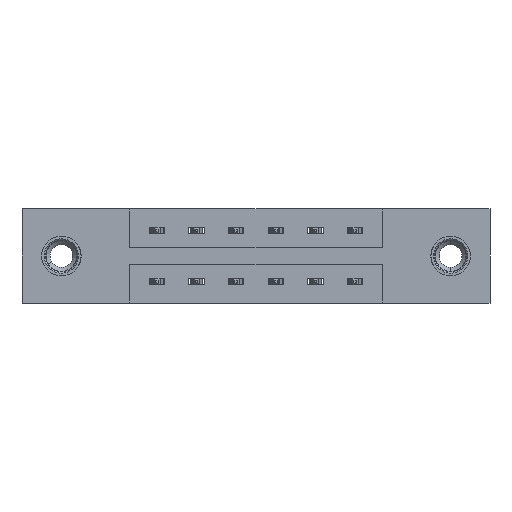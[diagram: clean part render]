
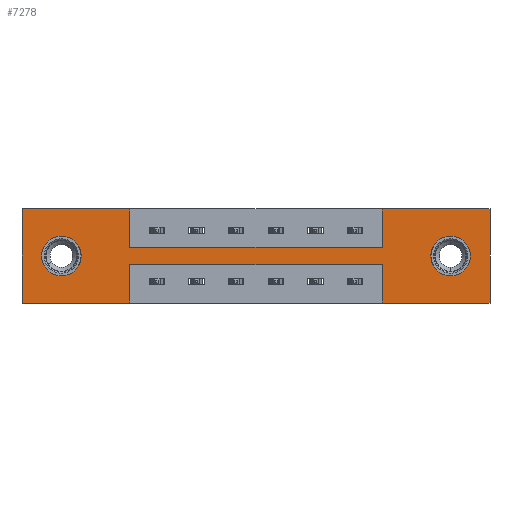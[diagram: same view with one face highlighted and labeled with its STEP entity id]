
A CAD part, front view. The second image highlights one B-rep face of the part: STEP entity #7278.
In plain terms, the highlighted planar face has unit normal (0, -1, 0).
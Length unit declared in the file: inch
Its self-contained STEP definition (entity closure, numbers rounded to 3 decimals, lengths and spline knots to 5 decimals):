
#63 = FACE_BOUND ( 'NONE', #5613, .T. ) ;
#370 = DIRECTION ( 'NONE',  ( 0., 0., 1. ) ) ;
#377 = DIRECTION ( 'NONE',  ( 0., 0., 1. ) ) ;
#444 = DIRECTION ( 'NONE',  ( 0., 0., 1. ) ) ;
#458 = CARTESIAN_POINT ( 'NONE',  ( 0., 0., 0. ) ) ;
#507 = DIRECTION ( 'NONE',  ( 0., 0., 1. ) ) ;
#726 = LINE ( 'NONE', #10218, #7876 ) ;
#745 = CARTESIAN_POINT ( 'NONE',  ( 0., 0., 0. ) ) ;
#850 = EDGE_CURVE ( 'NONE', #5885, #9751, #726, .T. ) ;
#932 = LINE ( 'NONE', #745, #8603 ) ;
#1276 = LINE ( 'NONE', #458, #6536 ) ;
#1487 = EDGE_LOOP ( 'NONE', ( #7969, #8581, #2194, #3082, #7238, #6173, #7760, #5779, #2649, #6108, #7598, #5105 ) ) ;
#1727 = DIRECTION ( 'NONE',  ( 0., 1., 0. ) ) ;
#1760 = DIRECTION ( 'NONE',  ( -1., 0., 0. ) ) ;
#1803 = CARTESIAN_POINT ( 'NONE',  ( 1.842, 0., -0.37 ) ) ;
#1879 = EDGE_CURVE ( 'NONE', #3260, #9909, #4144, .T. ) ;
#1984 = DIRECTION ( 'NONE',  ( 0., 0., -1. ) ) ;
#1999 = ORIENTED_EDGE ( 'NONE', *, *, #6703, .T. ) ;
#2004 = AXIS2_PLACEMENT_3D ( 'NONE', #3035, #6386, #4793 ) ;
#2066 = EDGE_CURVE ( 'NONE', #6498, #4784, #5661, .T. ) ;
#2078 = FACE_BOUND ( 'NONE', #5520, .T. ) ;
#2093 = DIRECTION ( 'NONE',  ( 0., 0., -1. ) ) ;
#2112 = VERTEX_POINT ( 'NONE', #7052 ) ;
#2194 = ORIENTED_EDGE ( 'NONE', *, *, #6583, .F. ) ;
#2346 = EDGE_CURVE ( 'NONE', #5500, #9208, #4010, .T. ) ;
#2453 = EDGE_CURVE ( 'NONE', #5859, #4353, #932, .T. ) ;
#2478 = LINE ( 'NONE', #4510, #4418 ) ;
#2520 = CARTESIAN_POINT ( 'NONE',  ( 1.417, 0., -0.22 ) ) ;
#2649 = ORIENTED_EDGE ( 'NONE', *, *, #8622, .F. ) ;
#2692 = DIRECTION ( 'NONE',  ( 0., 0., -1. ) ) ;
#2848 = DIRECTION ( 'NONE',  ( 0., 1., 0. ) ) ;
#3035 = CARTESIAN_POINT ( 'NONE',  ( 0.155, 0., -0.185 ) ) ;
#3072 = DIRECTION ( 'NONE',  ( 0., 1., 0. ) ) ;
#3082 = ORIENTED_EDGE ( 'NONE', *, *, #1879, .F. ) ;
#3260 = VERTEX_POINT ( 'NONE', #1803 ) ;
#3330 = CARTESIAN_POINT ( 'NONE',  ( 1.687, 0., -0.185 ) ) ;
#3487 = LINE ( 'NONE', #3675, #8743 ) ;
#3525 = CARTESIAN_POINT ( 'NONE',  ( 0.155, 0., -0.185 ) ) ;
#3571 = CARTESIAN_POINT ( 'NONE',  ( 0., 0., 0. ) ) ;
#3597 = CARTESIAN_POINT ( 'NONE',  ( 1.417, 0., -0.37 ) ) ;
#3664 = DIRECTION ( 'NONE',  ( 1., 0., 0. ) ) ;
#3675 = CARTESIAN_POINT ( 'NONE',  ( 1.417, 0., 0. ) ) ;
#3828 = DIRECTION ( 'NONE',  ( 0., 0., -1. ) ) ;
#3837 = CARTESIAN_POINT ( 'NONE',  ( 0.155, 0., -0.263 ) ) ;
#3886 = FACE_OUTER_BOUND ( 'NONE', #1487, .T. ) ;
#3925 = VERTEX_POINT ( 'NONE', #8525 ) ;
#3940 = EDGE_CURVE ( 'NONE', #8031, #3925, #1276, .T. ) ;
#4006 = VECTOR ( 'NONE', #6531, 39.37008 ) ;
#4010 = CIRCLE ( 'NONE', #5925, 0.078 ) ;
#4053 = CARTESIAN_POINT ( 'NONE',  ( 0.425, 0., -0.37 ) ) ;
#4144 = LINE ( 'NONE', #6759, #10363 ) ;
#4169 = CARTESIAN_POINT ( 'NONE',  ( 1.687, 0., -0.263 ) ) ;
#4216 = VECTOR ( 'NONE', #377, 39.37008 ) ;
#4353 = VERTEX_POINT ( 'NONE', #5082 ) ;
#4418 = VECTOR ( 'NONE', #2093, 39.37008 ) ;
#4470 = EDGE_CURVE ( 'NONE', #9751, #5859, #6525, .T. ) ;
#4497 = CARTESIAN_POINT ( 'NONE',  ( 0.425, 0., -0.22 ) ) ;
#4510 = CARTESIAN_POINT ( 'NONE',  ( 0.425, 0., -0.37 ) ) ;
#4784 = VERTEX_POINT ( 'NONE', #6751 ) ;
#4793 = DIRECTION ( 'NONE',  ( 0., 0., 1. ) ) ;
#5082 = CARTESIAN_POINT ( 'NONE',  ( 0.425, 0., 0. ) ) ;
#5105 = ORIENTED_EDGE ( 'NONE', *, *, #850, .F. ) ;
#5111 = DIRECTION ( 'NONE',  ( 1., 0., 0. ) ) ;
#5251 = CARTESIAN_POINT ( 'NONE',  ( 1.687, 0., -0.107 ) ) ;
#5297 = DIRECTION ( 'NONE',  ( -1., 0., 0. ) ) ;
#5389 = CARTESIAN_POINT ( 'NONE',  ( 0.425, 0., -0.15 ) ) ;
#5396 = DIRECTION ( 'NONE',  ( -1., 0., 0. ) ) ;
#5412 = LINE ( 'NONE', #7024, #7847 ) ;
#5500 = VERTEX_POINT ( 'NONE', #5251 ) ;
#5520 = EDGE_LOOP ( 'NONE', ( #7944, #1999 ) ) ;
#5613 = EDGE_LOOP ( 'NONE', ( #9435, #9003 ) ) ;
#5646 = CARTESIAN_POINT ( 'NONE',  ( 0., 0., 0. ) ) ;
#5661 = LINE ( 'NONE', #4497, #9735 ) ;
#5779 = ORIENTED_EDGE ( 'NONE', *, *, #6575, .F. ) ;
#5794 = VERTEX_POINT ( 'NONE', #3837 ) ;
#5810 = CARTESIAN_POINT ( 'NONE',  ( 0., 0., -0.37 ) ) ;
#5859 = VERTEX_POINT ( 'NONE', #5646 ) ;
#5885 = VERTEX_POINT ( 'NONE', #4053 ) ;
#5925 = AXIS2_PLACEMENT_3D ( 'NONE', #3330, #1727, #2692 ) ;
#6108 = ORIENTED_EDGE ( 'NONE', *, *, #2453, .F. ) ;
#6166 = AXIS2_PLACEMENT_3D ( 'NONE', #7216, #3072, #8852 ) ;
#6173 = ORIENTED_EDGE ( 'NONE', *, *, #3940, .F. ) ;
#6213 = LINE ( 'NONE', #9437, #9136 ) ;
#6254 = EDGE_CURVE ( 'NONE', #4784, #5885, #2478, .T. ) ;
#6333 = LINE ( 'NONE', #5389, #8882 ) ;
#6386 = DIRECTION ( 'NONE',  ( 0., 1., 0. ) ) ;
#6498 = VERTEX_POINT ( 'NONE', #2520 ) ;
#6525 = LINE ( 'NONE', #3571, #4216 ) ;
#6531 = DIRECTION ( 'NONE',  ( 0., 0., -1. ) ) ;
#6536 = VECTOR ( 'NONE', #10277, 39.37008 ) ;
#6575 = EDGE_CURVE ( 'NONE', #2112, #8388, #6333, .T. ) ;
#6583 = EDGE_CURVE ( 'NONE', #9909, #6498, #6213, .T. ) ;
#6703 = EDGE_CURVE ( 'NONE', #5794, #8820, #6734, .T. ) ;
#6734 = CIRCLE ( 'NONE', #2004, 0.078 ) ;
#6751 = CARTESIAN_POINT ( 'NONE',  ( 0.425, 0., -0.22 ) ) ;
#6759 = CARTESIAN_POINT ( 'NONE',  ( 0., 0., -0.37 ) ) ;
#7024 = CARTESIAN_POINT ( 'NONE',  ( 0.425, 0., 0. ) ) ;
#7052 = CARTESIAN_POINT ( 'NONE',  ( 0.425, 0., -0.15 ) ) ;
#7216 = CARTESIAN_POINT ( 'NONE',  ( 1.687, 0., -0.185 ) ) ;
#7238 = ORIENTED_EDGE ( 'NONE', *, *, #7986, .F. ) ;
#7278 = ADVANCED_FACE ( 'NONE', ( #63, #2078, #3886 ), #9481, .T. ) ;
#7297 = CIRCLE ( 'NONE', #6166, 0.078 ) ;
#7305 = LINE ( 'NONE', #9634, #4006 ) ;
#7502 = CARTESIAN_POINT ( 'NONE',  ( 0.155, 0., -0.107 ) ) ;
#7564 = EDGE_CURVE ( 'NONE', #8388, #8031, #3487, .T. ) ;
#7598 = ORIENTED_EDGE ( 'NONE', *, *, #4470, .F. ) ;
#7760 = ORIENTED_EDGE ( 'NONE', *, *, #7564, .F. ) ;
#7800 = AXIS2_PLACEMENT_3D ( 'NONE', #9427, #7917, #3828 ) ;
#7847 = VECTOR ( 'NONE', #1984, 39.37008 ) ;
#7872 = CARTESIAN_POINT ( 'NONE',  ( 1.417, 0., -0.15 ) ) ;
#7876 = VECTOR ( 'NONE', #5297, 39.37008 ) ;
#7917 = DIRECTION ( 'NONE',  ( 0., -1., 0. ) ) ;
#7944 = ORIENTED_EDGE ( 'NONE', *, *, #9924, .T. ) ;
#7969 = ORIENTED_EDGE ( 'NONE', *, *, #6254, .F. ) ;
#7986 = EDGE_CURVE ( 'NONE', #3925, #3260, #7305, .T. ) ;
#8031 = VERTEX_POINT ( 'NONE', #10506 ) ;
#8355 = AXIS2_PLACEMENT_3D ( 'NONE', #3525, #2848, #370 ) ;
#8388 = VERTEX_POINT ( 'NONE', #7872 ) ;
#8412 = CIRCLE ( 'NONE', #8355, 0.078 ) ;
#8525 = CARTESIAN_POINT ( 'NONE',  ( 1.842, 0., 0. ) ) ;
#8581 = ORIENTED_EDGE ( 'NONE', *, *, #2066, .F. ) ;
#8603 = VECTOR ( 'NONE', #5111, 39.37008 ) ;
#8622 = EDGE_CURVE ( 'NONE', #4353, #2112, #5412, .T. ) ;
#8743 = VECTOR ( 'NONE', #444, 39.37008 ) ;
#8820 = VERTEX_POINT ( 'NONE', #7502 ) ;
#8852 = DIRECTION ( 'NONE',  ( 0., 0., -1. ) ) ;
#8882 = VECTOR ( 'NONE', #3664, 39.37008 ) ;
#8994 = EDGE_CURVE ( 'NONE', #9208, #5500, #7297, .T. ) ;
#9003 = ORIENTED_EDGE ( 'NONE', *, *, #8994, .T. ) ;
#9136 = VECTOR ( 'NONE', #507, 39.37008 ) ;
#9208 = VERTEX_POINT ( 'NONE', #4169 ) ;
#9427 = CARTESIAN_POINT ( 'NONE',  ( 0., 0., -0.37 ) ) ;
#9435 = ORIENTED_EDGE ( 'NONE', *, *, #2346, .T. ) ;
#9437 = CARTESIAN_POINT ( 'NONE',  ( 1.417, 0., -0.37 ) ) ;
#9481 = PLANE ( 'NONE',  #7800 ) ;
#9634 = CARTESIAN_POINT ( 'NONE',  ( 1.842, 0., 0. ) ) ;
#9735 = VECTOR ( 'NONE', #5396, 39.37008 ) ;
#9751 = VERTEX_POINT ( 'NONE', #5810 ) ;
#9909 = VERTEX_POINT ( 'NONE', #3597 ) ;
#9924 = EDGE_CURVE ( 'NONE', #8820, #5794, #8412, .T. ) ;
#10218 = CARTESIAN_POINT ( 'NONE',  ( 0., 0., -0.37 ) ) ;
#10277 = DIRECTION ( 'NONE',  ( 1., 0., 0. ) ) ;
#10363 = VECTOR ( 'NONE', #1760, 39.37008 ) ;
#10506 = CARTESIAN_POINT ( 'NONE',  ( 1.417, 0., 0. ) ) ;
